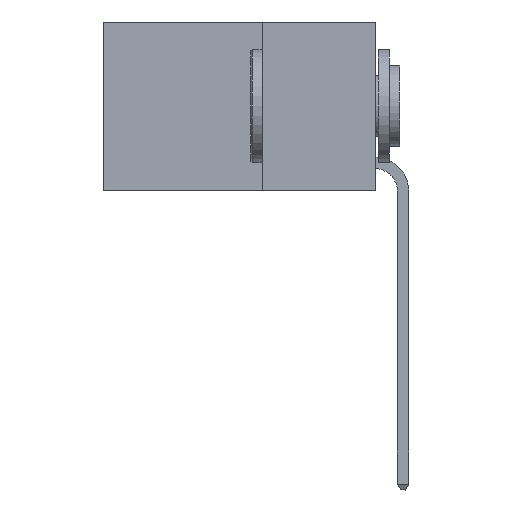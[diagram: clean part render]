
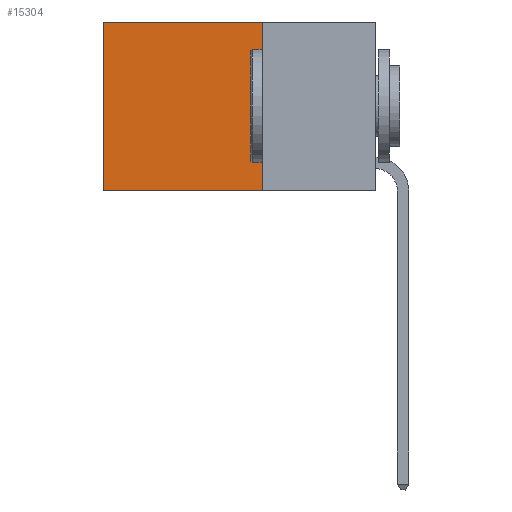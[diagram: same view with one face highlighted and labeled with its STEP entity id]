
A CAD part, left-side view. The second image highlights one B-rep face of the part: STEP entity #15304.
In plain terms, the highlighted planar face has unit normal (-1, 0, 0).
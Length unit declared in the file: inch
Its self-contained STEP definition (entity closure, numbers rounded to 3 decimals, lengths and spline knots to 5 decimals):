
#58 = DIRECTION ( 'NONE',  ( 0., 1., 0. ) ) ;
#539 = CARTESIAN_POINT ( 'NONE',  ( 0.2625, 0.6, -0.37 ) ) ;
#1677 = ORIENTED_EDGE ( 'NONE', *, *, #6353, .F. ) ;
#3160 = CARTESIAN_POINT ( 'NONE',  ( 0.2625, 0.25, 0. ) ) ;
#4161 = CARTESIAN_POINT ( 'NONE',  ( 0.2625, 0.6, 0. ) ) ;
#6353 = EDGE_CURVE ( 'NONE', #10503, #16091, #21301, .T. ) ;
#6658 = ORIENTED_EDGE ( 'NONE', *, *, #7316, .T. ) ;
#7316 = EDGE_CURVE ( 'NONE', #24341, #13519, #23533, .T. ) ;
#9306 = DIRECTION ( 'NONE',  ( 1., 0., 0. ) ) ;
#10503 = VERTEX_POINT ( 'NONE', #13579 ) ;
#12235 = AXIS2_PLACEMENT_3D ( 'NONE', #13791, #9306, #25340 ) ;
#13351 = EDGE_CURVE ( 'NONE', #24341, #10503, #19354, .T. ) ;
#13519 = VERTEX_POINT ( 'NONE', #4161 ) ;
#13579 = CARTESIAN_POINT ( 'NONE',  ( 0.2625, 0.25, -0.37 ) ) ;
#13791 = CARTESIAN_POINT ( 'NONE',  ( 0.2625, 0.25, 0. ) ) ;
#14607 = EDGE_CURVE ( 'NONE', #13519, #16091, #23846, .T. ) ;
#15304 = ADVANCED_FACE ( 'NONE', ( #22734 ), #20727, .F. ) ;
#15930 = ORIENTED_EDGE ( 'NONE', *, *, #14607, .T. ) ;
#16091 = VERTEX_POINT ( 'NONE', #539 ) ;
#16198 = CARTESIAN_POINT ( 'NONE',  ( 0.2625, 0.25, -0.37 ) ) ;
#17162 = DIRECTION ( 'NONE',  ( 0., 0., -1. ) ) ;
#18634 = VECTOR ( 'NONE', #28790, 39.37008 ) ;
#18684 = EDGE_LOOP ( 'NONE', ( #15930, #1677, #22301, #6658 ) ) ;
#19354 = LINE ( 'NONE', #26443, #18634 ) ;
#19593 = DIRECTION ( 'NONE',  ( 0., 1., 0. ) ) ;
#20727 = PLANE ( 'NONE',  #12235 ) ;
#21301 = LINE ( 'NONE', #16198, #26667 ) ;
#22301 = ORIENTED_EDGE ( 'NONE', *, *, #13351, .F. ) ;
#22734 = FACE_OUTER_BOUND ( 'NONE', #18684, .T. ) ;
#23533 = LINE ( 'NONE', #26365, #23764 ) ;
#23764 = VECTOR ( 'NONE', #19593, 39.37008 ) ;
#23846 = LINE ( 'NONE', #28529, #29136 ) ;
#24341 = VERTEX_POINT ( 'NONE', #3160 ) ;
#25340 = DIRECTION ( 'NONE',  ( 0., 0., -1. ) ) ;
#26365 = CARTESIAN_POINT ( 'NONE',  ( 0.2625, 0.25, 0. ) ) ;
#26443 = CARTESIAN_POINT ( 'NONE',  ( 0.2625, 0.25, 0. ) ) ;
#26667 = VECTOR ( 'NONE', #58, 39.37008 ) ;
#28529 = CARTESIAN_POINT ( 'NONE',  ( 0.2625, 0.6, 0. ) ) ;
#28790 = DIRECTION ( 'NONE',  ( 0., 0., -1. ) ) ;
#29136 = VECTOR ( 'NONE', #17162, 39.37008 ) ;
